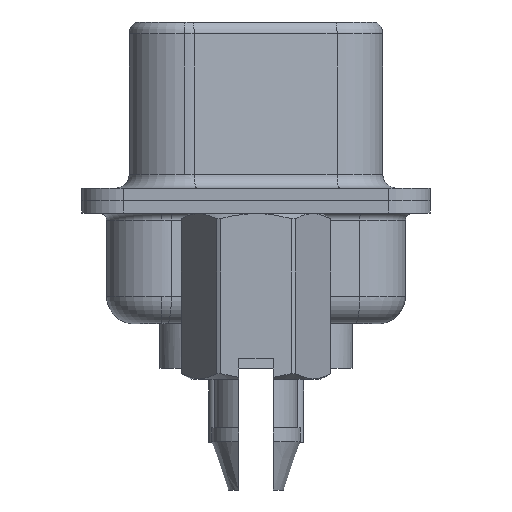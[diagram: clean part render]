
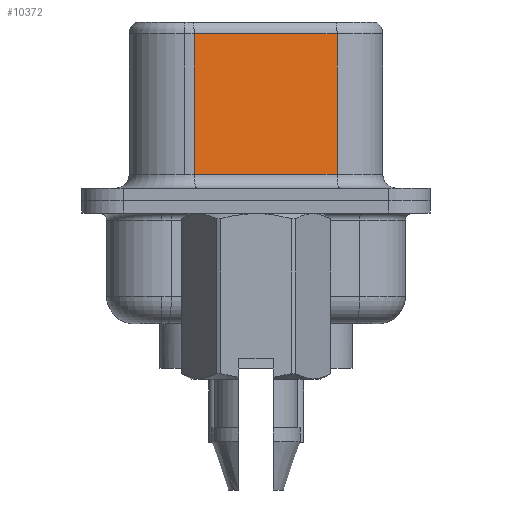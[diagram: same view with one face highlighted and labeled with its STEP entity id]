
A CAD part, left-side view. The second image highlights one B-rep face of the part: STEP entity #10372.
In plain terms, the highlighted planar face has unit normal (-0.985, -0.174, 0).
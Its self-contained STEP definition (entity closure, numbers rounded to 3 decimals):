
#964 = CARTESIAN_POINT ( 'NONE',  ( 4.58, -2.927, 6.02 ) ) ;
#2345 = LINE ( 'NONE', #10173, #13145 ) ;
#2567 = VECTOR ( 'NONE', #15197, 1000. ) ;
#4182 = AXIS2_PLACEMENT_3D ( 'NONE', #10772, #24965, #12837 ) ;
#5423 = CARTESIAN_POINT ( 'NONE',  ( 4.58, -2.927, 6.02 ) ) ;
#5999 = CARTESIAN_POINT ( 'NONE',  ( 4.58, -2.927, 6.52 ) ) ;
#6453 = ORIENTED_EDGE ( 'NONE', *, *, #12108, .F. ) ;
#7920 = LINE ( 'NONE', #964, #2567 ) ;
#7954 = ORIENTED_EDGE ( 'NONE', *, *, #18914, .T. ) ;
#8314 = LINE ( 'NONE', #24182, #8964 ) ;
#8964 = VECTOR ( 'NONE', #12072, 1000. ) ;
#9132 = VERTEX_POINT ( 'NONE', #5423 ) ;
#9653 = CARTESIAN_POINT ( 'NONE',  ( 3.67, 2.233, 6.02 ) ) ;
#10173 = CARTESIAN_POINT ( 'NONE',  ( 4.58, -2.927, 0.95 ) ) ;
#10189 = CARTESIAN_POINT ( 'NONE',  ( 3.67, 2.233, 0.95 ) ) ;
#10372 = ADVANCED_FACE ( 'NONE', ( #19290 ), #16815, .F. ) ;
#10691 = LINE ( 'NONE', #5999, #20764 ) ;
#10772 = CARTESIAN_POINT ( 'NONE',  ( 4.58, -2.927, 6.52 ) ) ;
#11401 = EDGE_LOOP ( 'NONE', ( #6453, #7954, #11634, #17828 ) ) ;
#11634 = ORIENTED_EDGE ( 'NONE', *, *, #14031, .T. ) ;
#12072 = DIRECTION ( 'NONE',  ( 0., 0., -1. ) ) ;
#12108 = EDGE_CURVE ( 'NONE', #9132, #16937, #10691, .T. ) ;
#12837 = DIRECTION ( 'NONE',  ( -0.174, 0.985, 0. ) ) ;
#13145 = VECTOR ( 'NONE', #24389, 1000. ) ;
#14031 = EDGE_CURVE ( 'NONE', #21876, #15059, #8314, .T. ) ;
#14375 = CARTESIAN_POINT ( 'NONE',  ( 4.58, -2.927, 0.95 ) ) ;
#14829 = EDGE_CURVE ( 'NONE', #15059, #16937, #2345, .T. ) ;
#15059 = VERTEX_POINT ( 'NONE', #10189 ) ;
#15197 = DIRECTION ( 'NONE',  ( -0.174, 0.985, 0. ) ) ;
#16815 = PLANE ( 'NONE',  #4182 ) ;
#16937 = VERTEX_POINT ( 'NONE', #14375 ) ;
#17828 = ORIENTED_EDGE ( 'NONE', *, *, #14829, .T. ) ;
#18251 = DIRECTION ( 'NONE',  ( 0., 0., -1. ) ) ;
#18914 = EDGE_CURVE ( 'NONE', #9132, #21876, #7920, .T. ) ;
#19290 = FACE_OUTER_BOUND ( 'NONE', #11401, .T. ) ;
#20764 = VECTOR ( 'NONE', #18251, 1000. ) ;
#21876 = VERTEX_POINT ( 'NONE', #9653 ) ;
#24182 = CARTESIAN_POINT ( 'NONE',  ( 3.67, 2.233, 6.52 ) ) ;
#24389 = DIRECTION ( 'NONE',  ( 0.174, -0.985, 0. ) ) ;
#24965 = DIRECTION ( 'NONE',  ( 0.985, 0.174, 0. ) ) ;
